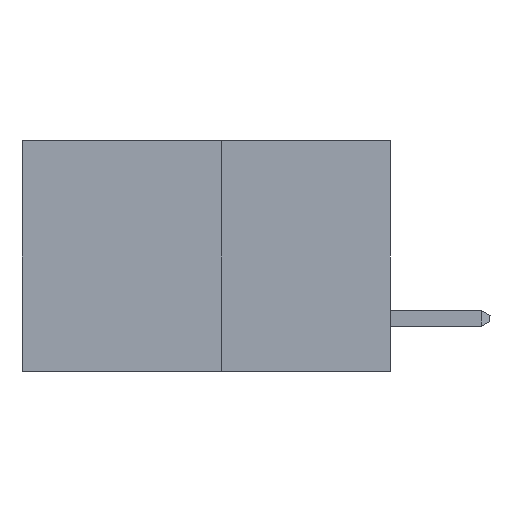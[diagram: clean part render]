
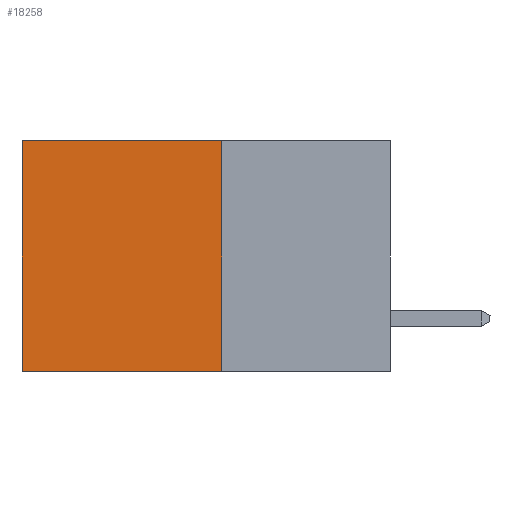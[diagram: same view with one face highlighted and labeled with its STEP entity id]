
A CAD part, left-side view. The second image highlights one B-rep face of the part: STEP entity #18258.
In plain terms, the highlighted planar face has unit normal (-1, 0, 0).
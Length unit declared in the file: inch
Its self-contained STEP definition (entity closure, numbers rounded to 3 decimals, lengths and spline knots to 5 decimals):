
#1269 = CARTESIAN_POINT ( 'NONE',  ( 0.277, 0.27, -0.37 ) ) ;
#2748 = DIRECTION ( 'NONE',  ( 0., 0., -1. ) ) ;
#3315 = EDGE_CURVE ( 'NONE', #7721, #12392, #18859, .T. ) ;
#3641 = LINE ( 'NONE', #10998, #14954 ) ;
#4544 = DIRECTION ( 'NONE',  ( 0., 1., 0. ) ) ;
#4567 = CARTESIAN_POINT ( 'NONE',  ( 0.277, 0.59, 0. ) ) ;
#4874 = VERTEX_POINT ( 'NONE', #10252 ) ;
#6921 = VECTOR ( 'NONE', #8000, 39.37008 ) ;
#7041 = FACE_OUTER_BOUND ( 'NONE', #10318, .T. ) ;
#7176 = CARTESIAN_POINT ( 'NONE',  ( 0.277, 0.59, -0.37 ) ) ;
#7193 = PLANE ( 'NONE',  #9360 ) ;
#7319 = VECTOR ( 'NONE', #4544, 39.37008 ) ;
#7721 = VERTEX_POINT ( 'NONE', #18458 ) ;
#8000 = DIRECTION ( 'NONE',  ( 0., 0., -1. ) ) ;
#8033 = DIRECTION ( 'NONE',  ( 0., 1., 0. ) ) ;
#8114 = ORIENTED_EDGE ( 'NONE', *, *, #3315, .F. ) ;
#9236 = VECTOR ( 'NONE', #17738, 39.37008 ) ;
#9360 = AXIS2_PLACEMENT_3D ( 'NONE', #1269, #11736, #2748 ) ;
#10252 = CARTESIAN_POINT ( 'NONE',  ( 0.277, 0.59, -0.37 ) ) ;
#10295 = EDGE_CURVE ( 'NONE', #12392, #4874, #19231, .T. ) ;
#10318 = EDGE_LOOP ( 'NONE', ( #17296, #17251, #8114, #15392 ) ) ;
#10998 = CARTESIAN_POINT ( 'NONE',  ( 0.277, 0.27, 0. ) ) ;
#11736 = DIRECTION ( 'NONE',  ( 1., 0., 0. ) ) ;
#12392 = VERTEX_POINT ( 'NONE', #12840 ) ;
#12840 = CARTESIAN_POINT ( 'NONE',  ( 0.277, 0.27, -0.37 ) ) ;
#13772 = LINE ( 'NONE', #7176, #9236 ) ;
#14639 = CARTESIAN_POINT ( 'NONE',  ( 0.277, 0.27, -0.37 ) ) ;
#14780 = VERTEX_POINT ( 'NONE', #4567 ) ;
#14954 = VECTOR ( 'NONE', #8033, 39.37008 ) ;
#15053 = CARTESIAN_POINT ( 'NONE',  ( 0.277, 0.27, -0.37 ) ) ;
#15392 = ORIENTED_EDGE ( 'NONE', *, *, #16589, .T. ) ;
#16589 = EDGE_CURVE ( 'NONE', #7721, #14780, #3641, .T. ) ;
#16904 = EDGE_CURVE ( 'NONE', #14780, #4874, #13772, .T. ) ;
#17251 = ORIENTED_EDGE ( 'NONE', *, *, #10295, .F. ) ;
#17296 = ORIENTED_EDGE ( 'NONE', *, *, #16904, .T. ) ;
#17738 = DIRECTION ( 'NONE',  ( 0., 0., -1. ) ) ;
#18258 = ADVANCED_FACE ( 'NONE', ( #7041 ), #7193, .F. ) ;
#18458 = CARTESIAN_POINT ( 'NONE',  ( 0.277, 0.27, 0. ) ) ;
#18859 = LINE ( 'NONE', #14639, #6921 ) ;
#19231 = LINE ( 'NONE', #15053, #7319 ) ;
